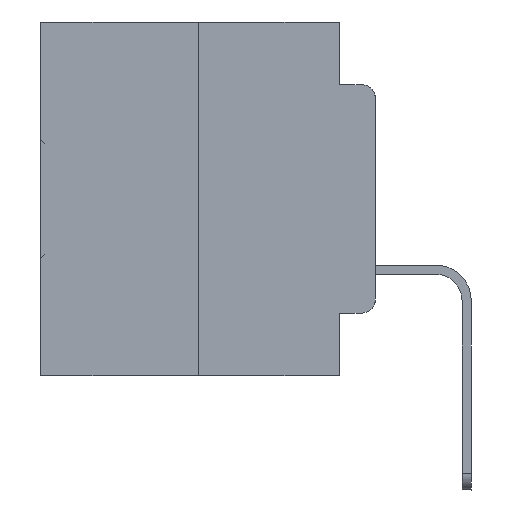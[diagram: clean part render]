
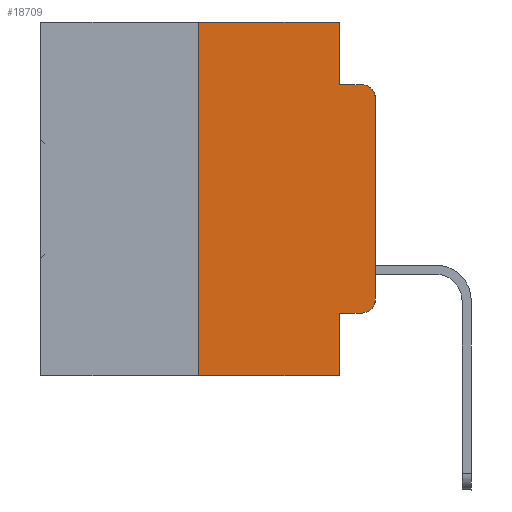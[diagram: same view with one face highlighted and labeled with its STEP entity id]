
A CAD part, left-side view. The second image highlights one B-rep face of the part: STEP entity #18709.
In plain terms, the highlighted planar face has unit normal (-1, 0, 0).
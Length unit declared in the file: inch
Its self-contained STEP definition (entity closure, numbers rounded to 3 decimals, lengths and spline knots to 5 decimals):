
#82 = VECTOR ( 'NONE', #7153, 39.37008 ) ;
#767 = DIRECTION ( 'NONE',  ( 0., 0., -1. ) ) ;
#2403 = VERTEX_POINT ( 'NONE', #5622 ) ;
#2687 = DIRECTION ( 'NONE',  ( 0., 0., -1. ) ) ;
#2804 = CIRCLE ( 'NONE', #14533, 0.02 ) ;
#3342 = ORIENTED_EDGE ( 'NONE', *, *, #18317, .T. ) ;
#4062 = CARTESIAN_POINT ( 'NONE',  ( 0., 0.051, 0. ) ) ;
#4744 = CARTESIAN_POINT ( 'NONE',  ( 0., 0.473, 0. ) ) ;
#5101 = VERTEX_POINT ( 'NONE', #29916 ) ;
#5322 = EDGE_CURVE ( 'NONE', #12115, #5101, #2804, .T. ) ;
#5588 = VERTEX_POINT ( 'NONE', #16275 ) ;
#5622 = CARTESIAN_POINT ( 'NONE',  ( 0., 0.02, -0.4115 ) ) ;
#5720 = VECTOR ( 'NONE', #27287, 39.37008 ) ;
#5751 = LINE ( 'NONE', #14569, #5720 ) ;
#6075 = VERTEX_POINT ( 'NONE', #31061 ) ;
#6395 = EDGE_CURVE ( 'NONE', #30746, #5588, #22245, .T. ) ;
#6461 = CARTESIAN_POINT ( 'NONE',  ( 0., 0.25, 0. ) ) ;
#7153 = DIRECTION ( 'NONE',  ( 0., 0., -1. ) ) ;
#7360 = VERTEX_POINT ( 'NONE', #22709 ) ;
#7849 = DIRECTION ( 'NONE',  ( 0., -1., 0. ) ) ;
#8078 = EDGE_CURVE ( 'NONE', #26571, #2403, #28478, .T. ) ;
#8382 = EDGE_CURVE ( 'NONE', #11359, #30746, #18566, .T. ) ;
#8540 = ORIENTED_EDGE ( 'NONE', *, *, #5322, .T. ) ;
#9872 = VECTOR ( 'NONE', #19535, 39.37008 ) ;
#10277 = FACE_OUTER_BOUND ( 'NONE', #12543, .T. ) ;
#10415 = ORIENTED_EDGE ( 'NONE', *, *, #11670, .F. ) ;
#10863 = CARTESIAN_POINT ( 'NONE',  ( 0., 0., 0. ) ) ;
#10904 = CARTESIAN_POINT ( 'NONE',  ( 0., 0.473, 0. ) ) ;
#10989 = DIRECTION ( 'NONE',  ( 0., 0., -1. ) ) ;
#11359 = VERTEX_POINT ( 'NONE', #18598 ) ;
#11507 = VECTOR ( 'NONE', #28656, 39.37008 ) ;
#11670 = EDGE_CURVE ( 'NONE', #5588, #7360, #28609, .T. ) ;
#12115 = VERTEX_POINT ( 'NONE', #22268 ) ;
#12543 = EDGE_LOOP ( 'NONE', ( #3342, #8540, #22965, #10415, #15895, #23488, #23458, #15133, #26911, #13478 ) ) ;
#12693 = LINE ( 'NONE', #28794, #15866 ) ;
#12700 = EDGE_CURVE ( 'NONE', #11359, #6075, #5751, .T. ) ;
#13284 = CARTESIAN_POINT ( 'NONE',  ( 0., 0.02, -0.3915 ) ) ;
#13478 = ORIENTED_EDGE ( 'NONE', *, *, #29814, .T. ) ;
#14533 = AXIS2_PLACEMENT_3D ( 'NONE', #20294, #15303, #2687 ) ;
#14569 = CARTESIAN_POINT ( 'NONE',  ( 0., 0.473, -0.5 ) ) ;
#15133 = ORIENTED_EDGE ( 'NONE', *, *, #23272, .F. ) ;
#15303 = DIRECTION ( 'NONE',  ( -1., 0., 0. ) ) ;
#15866 = VECTOR ( 'NONE', #10989, 39.37008 ) ;
#15895 = ORIENTED_EDGE ( 'NONE', *, *, #6395, .F. ) ;
#16273 = DIRECTION ( 'NONE',  ( -1., 0., 0. ) ) ;
#16275 = CARTESIAN_POINT ( 'NONE',  ( 0., 0.051, 0. ) ) ;
#17460 = CARTESIAN_POINT ( 'NONE',  ( 0., 0., -0.3915 ) ) ;
#17667 = CARTESIAN_POINT ( 'NONE',  ( 0., 0.051, -0.4115 ) ) ;
#18240 = LINE ( 'NONE', #10863, #11507 ) ;
#18317 = EDGE_CURVE ( 'NONE', #24874, #12115, #18240, .T. ) ;
#18566 = LINE ( 'NONE', #6461, #9872 ) ;
#18598 = CARTESIAN_POINT ( 'NONE',  ( 0., 0.25, -0.5 ) ) ;
#18709 = ADVANCED_FACE ( 'NONE', ( #10277 ), #19926, .F. ) ;
#19535 = DIRECTION ( 'NONE',  ( 0., 0., 1. ) ) ;
#19601 = CARTESIAN_POINT ( 'NONE',  ( 0., 0.051, -0.4115 ) ) ;
#19926 = PLANE ( 'NONE',  #24201 ) ;
#20294 = CARTESIAN_POINT ( 'NONE',  ( 0., 0.02, -0.1085 ) ) ;
#20739 = LINE ( 'NONE', #22816, #23496 ) ;
#21825 = EDGE_CURVE ( 'NONE', #7360, #5101, #20739, .T. ) ;
#22245 = LINE ( 'NONE', #10904, #27756 ) ;
#22268 = CARTESIAN_POINT ( 'NONE',  ( 0., 0., -0.1085 ) ) ;
#22709 = CARTESIAN_POINT ( 'NONE',  ( 0., 0.051, -0.0885 ) ) ;
#22816 = CARTESIAN_POINT ( 'NONE',  ( 0., 0.051, -0.0885 ) ) ;
#22965 = ORIENTED_EDGE ( 'NONE', *, *, #21825, .F. ) ;
#23272 = EDGE_CURVE ( 'NONE', #26571, #6075, #12693, .T. ) ;
#23458 = ORIENTED_EDGE ( 'NONE', *, *, #12700, .T. ) ;
#23488 = ORIENTED_EDGE ( 'NONE', *, *, #8382, .F. ) ;
#23496 = VECTOR ( 'NONE', #7849, 39.37008 ) ;
#24201 = AXIS2_PLACEMENT_3D ( 'NONE', #4744, #30315, #27979 ) ;
#24874 = VERTEX_POINT ( 'NONE', #17460 ) ;
#24878 = CARTESIAN_POINT ( 'NONE',  ( 0., 0.25, 0. ) ) ;
#26571 = VERTEX_POINT ( 'NONE', #19601 ) ;
#26911 = ORIENTED_EDGE ( 'NONE', *, *, #8078, .T. ) ;
#27287 = DIRECTION ( 'NONE',  ( 0., -1., 0. ) ) ;
#27698 = VECTOR ( 'NONE', #28596, 39.37008 ) ;
#27756 = VECTOR ( 'NONE', #28703, 39.37008 ) ;
#27979 = DIRECTION ( 'NONE',  ( 0., 0., -1. ) ) ;
#28478 = LINE ( 'NONE', #17667, #27698 ) ;
#28596 = DIRECTION ( 'NONE',  ( 0., -1., 0. ) ) ;
#28609 = LINE ( 'NONE', #4062, #82 ) ;
#28656 = DIRECTION ( 'NONE',  ( 0., 0., 1. ) ) ;
#28703 = DIRECTION ( 'NONE',  ( 0., -1., 0. ) ) ;
#28794 = CARTESIAN_POINT ( 'NONE',  ( 0., 0.051, 0. ) ) ;
#29814 = EDGE_CURVE ( 'NONE', #2403, #24874, #32156, .T. ) ;
#29916 = CARTESIAN_POINT ( 'NONE',  ( 0., 0.02, -0.0885 ) ) ;
#30315 = DIRECTION ( 'NONE',  ( 1., 0., 0. ) ) ;
#30746 = VERTEX_POINT ( 'NONE', #24878 ) ;
#31061 = CARTESIAN_POINT ( 'NONE',  ( 0., 0.051, -0.5 ) ) ;
#31219 = AXIS2_PLACEMENT_3D ( 'NONE', #13284, #16273, #767 ) ;
#32156 = CIRCLE ( 'NONE', #31219, 0.02 ) ;
